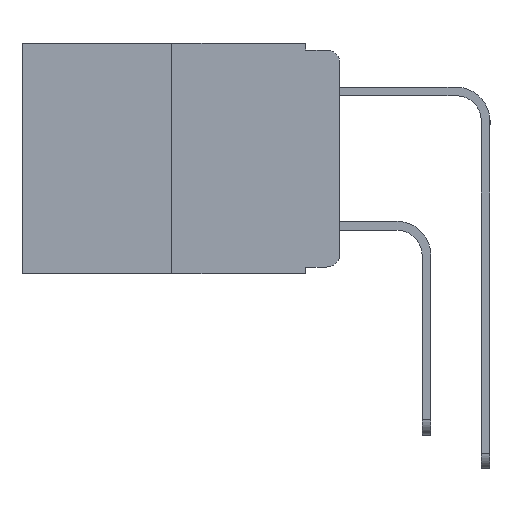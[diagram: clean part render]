
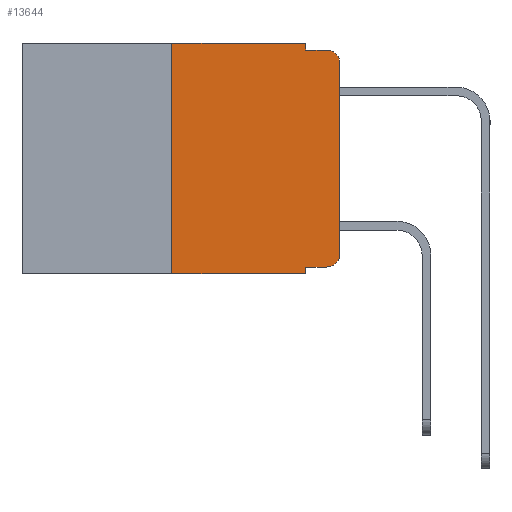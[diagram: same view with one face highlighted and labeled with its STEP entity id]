
A CAD part, left-side view. The second image highlights one B-rep face of the part: STEP entity #13644.
In plain terms, the highlighted planar face has unit normal (-1, 0, 0).
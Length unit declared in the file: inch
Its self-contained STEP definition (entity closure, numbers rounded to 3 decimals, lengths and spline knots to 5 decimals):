
#160 = ORIENTED_EDGE ( 'NONE', *, *, #9005, .T. ) ;
#229 = EDGE_CURVE ( 'NONE', #3835, #5821, #1881, .T. ) ;
#230 = CARTESIAN_POINT ( 'NONE',  ( 0., 0.473, -0.343 ) ) ;
#772 = ORIENTED_EDGE ( 'NONE', *, *, #8825, .T. ) ;
#1211 = CARTESIAN_POINT ( 'NONE',  ( 0., 0.051, -0.333 ) ) ;
#1355 = VERTEX_POINT ( 'NONE', #7717 ) ;
#1645 = DIRECTION ( 'NONE',  ( 0., -1., 0. ) ) ;
#1730 = CARTESIAN_POINT ( 'NONE',  ( 0., 0.473, 0. ) ) ;
#1749 = EDGE_CURVE ( 'NONE', #13958, #5821, #5230, .T. ) ;
#1881 = LINE ( 'NONE', #8856, #7510 ) ;
#2356 = DIRECTION ( 'NONE',  ( 0., 0., -1. ) ) ;
#2416 = ORIENTED_EDGE ( 'NONE', *, *, #13928, .F. ) ;
#2499 = EDGE_CURVE ( 'NONE', #9532, #13958, #7633, .T. ) ;
#2513 = DIRECTION ( 'NONE',  ( 0., 0., -1. ) ) ;
#2526 = ORIENTED_EDGE ( 'NONE', *, *, #1749, .T. ) ;
#2863 = DIRECTION ( 'NONE',  ( 0., 0., -1. ) ) ;
#3107 = CARTESIAN_POINT ( 'NONE',  ( 0., 0.02, -0.313 ) ) ;
#3835 = VERTEX_POINT ( 'NONE', #8222 ) ;
#4031 = AXIS2_PLACEMENT_3D ( 'NONE', #3107, #10903, #4222 ) ;
#4195 = LINE ( 'NONE', #8129, #9792 ) ;
#4221 = ORIENTED_EDGE ( 'NONE', *, *, #10269, .F. ) ;
#4222 = DIRECTION ( 'NONE',  ( 0., 0., -1. ) ) ;
#5230 = CIRCLE ( 'NONE', #13081, 0.02 ) ;
#5273 = LINE ( 'NONE', #6151, #7529 ) ;
#5446 = DIRECTION ( 'NONE',  ( -1., 0., 0. ) ) ;
#5715 = CARTESIAN_POINT ( 'NONE',  ( 0., 0.051, 0. ) ) ;
#5821 = VERTEX_POINT ( 'NONE', #9333 ) ;
#5868 = DIRECTION ( 'NONE',  ( 0., -1., 0. ) ) ;
#6151 = CARTESIAN_POINT ( 'NONE',  ( 0., 0.473, 0. ) ) ;
#6822 = CARTESIAN_POINT ( 'NONE',  ( 0., 0., -0.313 ) ) ;
#7020 = VECTOR ( 'NONE', #13394, 39.37008 ) ;
#7098 = LINE ( 'NONE', #8029, #9368 ) ;
#7332 = ORIENTED_EDGE ( 'NONE', *, *, #11747, .F. ) ;
#7376 = LINE ( 'NONE', #1211, #7020 ) ;
#7510 = VECTOR ( 'NONE', #10811, 39.37008 ) ;
#7529 = VECTOR ( 'NONE', #1645, 39.37008 ) ;
#7539 = ORIENTED_EDGE ( 'NONE', *, *, #9542, .T. ) ;
#7633 = LINE ( 'NONE', #12231, #10227 ) ;
#7638 = FACE_OUTER_BOUND ( 'NONE', #7738, .T. ) ;
#7717 = CARTESIAN_POINT ( 'NONE',  ( 0., 0.051, -0.343 ) ) ;
#7738 = EDGE_LOOP ( 'NONE', ( #12127, #2526, #11038, #2416, #8012, #7332, #160, #4221, #7539, #772 ) ) ;
#7885 = CARTESIAN_POINT ( 'NONE',  ( 0., 0.051, -0.333 ) ) ;
#8012 = ORIENTED_EDGE ( 'NONE', *, *, #10665, .F. ) ;
#8029 = CARTESIAN_POINT ( 'NONE',  ( 0., 0.051, 0. ) ) ;
#8129 = CARTESIAN_POINT ( 'NONE',  ( 0., 0.051, 0. ) ) ;
#8222 = CARTESIAN_POINT ( 'NONE',  ( 0., 0.051, -0.01 ) ) ;
#8238 = VECTOR ( 'NONE', #13750, 39.37008 ) ;
#8369 = VERTEX_POINT ( 'NONE', #7885 ) ;
#8483 = PLANE ( 'NONE',  #9787 ) ;
#8501 = VERTEX_POINT ( 'NONE', #9242 ) ;
#8819 = LINE ( 'NONE', #230, #11376 ) ;
#8825 = EDGE_CURVE ( 'NONE', #10349, #9532, #11214, .T. ) ;
#8856 = CARTESIAN_POINT ( 'NONE',  ( 0., 0.051, -0.01 ) ) ;
#9005 = EDGE_CURVE ( 'NONE', #8501, #1355, #8819, .T. ) ;
#9188 = CARTESIAN_POINT ( 'NONE',  ( 0., 0., -0.03 ) ) ;
#9242 = CARTESIAN_POINT ( 'NONE',  ( 0., 0.25, -0.343 ) ) ;
#9333 = CARTESIAN_POINT ( 'NONE',  ( 0., 0.02, -0.01 ) ) ;
#9368 = VECTOR ( 'NONE', #2356, 39.37008 ) ;
#9430 = CARTESIAN_POINT ( 'NONE',  ( 0., 0.02, -0.333 ) ) ;
#9532 = VERTEX_POINT ( 'NONE', #6822 ) ;
#9542 = EDGE_CURVE ( 'NONE', #8369, #10349, #7376, .T. ) ;
#9576 = DIRECTION ( 'NONE',  ( 1., 0., 0. ) ) ;
#9787 = AXIS2_PLACEMENT_3D ( 'NONE', #1730, #9576, #2863 ) ;
#9792 = VECTOR ( 'NONE', #2513, 39.37008 ) ;
#10227 = VECTOR ( 'NONE', #11131, 39.37008 ) ;
#10269 = EDGE_CURVE ( 'NONE', #8369, #1355, #4195, .T. ) ;
#10349 = VERTEX_POINT ( 'NONE', #9430 ) ;
#10473 = CARTESIAN_POINT ( 'NONE',  ( 0., 0.25, 0. ) ) ;
#10665 = EDGE_CURVE ( 'NONE', #11154, #12156, #5273, .T. ) ;
#10811 = DIRECTION ( 'NONE',  ( 0., -1., 0. ) ) ;
#10903 = DIRECTION ( 'NONE',  ( -1., 0., 0. ) ) ;
#11038 = ORIENTED_EDGE ( 'NONE', *, *, #229, .F. ) ;
#11131 = DIRECTION ( 'NONE',  ( 0., 0., 1. ) ) ;
#11154 = VERTEX_POINT ( 'NONE', #12534 ) ;
#11214 = CIRCLE ( 'NONE', #4031, 0.02 ) ;
#11376 = VECTOR ( 'NONE', #5868, 39.37008 ) ;
#11747 = EDGE_CURVE ( 'NONE', #8501, #11154, #14037, .T. ) ;
#12047 = CARTESIAN_POINT ( 'NONE',  ( 0., 0.02, -0.03 ) ) ;
#12127 = ORIENTED_EDGE ( 'NONE', *, *, #2499, .T. ) ;
#12156 = VERTEX_POINT ( 'NONE', #5715 ) ;
#12231 = CARTESIAN_POINT ( 'NONE',  ( 0., 0., 0. ) ) ;
#12534 = CARTESIAN_POINT ( 'NONE',  ( 0., 0.25, 0. ) ) ;
#13081 = AXIS2_PLACEMENT_3D ( 'NONE', #12047, #5446, #13148 ) ;
#13148 = DIRECTION ( 'NONE',  ( 0., 0., -1. ) ) ;
#13394 = DIRECTION ( 'NONE',  ( 0., -1., 0. ) ) ;
#13644 = ADVANCED_FACE ( 'NONE', ( #7638 ), #8483, .F. ) ;
#13750 = DIRECTION ( 'NONE',  ( 0., 0., 1. ) ) ;
#13928 = EDGE_CURVE ( 'NONE', #12156, #3835, #7098, .T. ) ;
#13958 = VERTEX_POINT ( 'NONE', #9188 ) ;
#14037 = LINE ( 'NONE', #10473, #8238 ) ;
